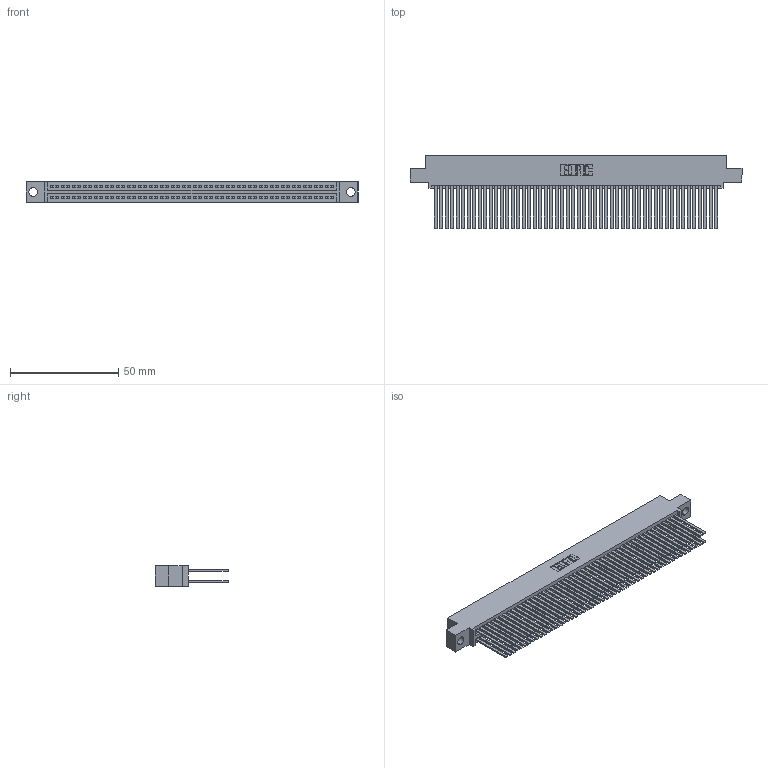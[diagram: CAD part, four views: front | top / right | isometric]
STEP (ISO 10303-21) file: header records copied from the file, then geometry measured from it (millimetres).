
FILE_DESCRIPTION (( 'STEP AP203' ), '1' );
FILE_NAME ('395-104-544-504.STEP', '2021-06-17T16:09:30', ( '' ), ( '' ), 'SwSTEP 2.0', 'SolidWorks 2020', '' );
FILE_SCHEMA (( 'CONFIG_CONTROL_DESIGN' ));
Length unit declared in the file: inch
Products named in the file (3): 345-292-001_345-293-144; 395-104-544-504; 345 Part_0.110 Offset - 0.156 Dia-TI
Assembly tree (105 placements, depth 2):
  395-104-544-504
    345 Part_0.110 Offset - 0.156 Dia-TI
    345-292-001_345-293-144  x104
Bounding box: 153.29 x 33.96 x 9.4 mm (x, y, z)
Volume: 16262 mm3; surface area: 28449.1 mm2
Topology: 105 solids, 105 shells, 4720 faces, 14013 edges, 9202 vertices
Faces by surface type: plane 3114, cylinder 1606
Entity records: 39821 total; most frequent: CARTESIAN_POINT 6670, ORIENTED_EDGE 6602, DIRECTION 5865, EDGE_CURVE 3301, LINE 2965, VECTOR 2965, VERTEX_POINT 2198, AXIS2_PLACEMENT_3D 1450
